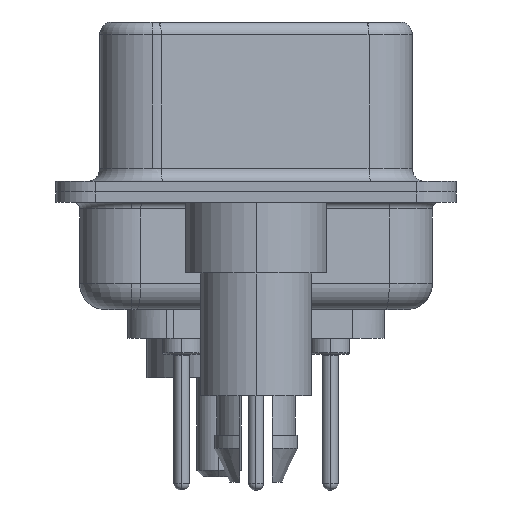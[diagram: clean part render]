
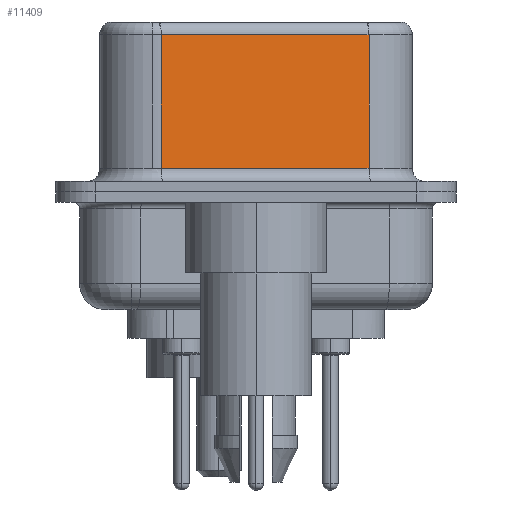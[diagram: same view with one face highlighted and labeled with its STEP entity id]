
A CAD part, left-side view. The second image highlights one B-rep face of the part: STEP entity #11409.
In plain terms, the highlighted planar face has unit normal (-0.985, -0.174, 0).
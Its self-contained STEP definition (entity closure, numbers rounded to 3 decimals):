
#6 = CARTESIAN_POINT ( 'NONE',  ( 5.132, -4.322, 6.02 ) ) ;
#261 = VECTOR ( 'NONE', #24384, 1000. ) ;
#1304 = EDGE_CURVE ( 'NONE', #33353, #19274, #29331, .T. ) ;
#1372 = EDGE_CURVE ( 'NONE', #15415, #19274, #7924, .T. ) ;
#1463 = DIRECTION ( 'NONE',  ( -0.174, 0.985, 0. ) ) ;
#1785 = CARTESIAN_POINT ( 'NONE',  ( 5.132, -4.322, 6.02 ) ) ;
#2035 = VERTEX_POINT ( 'NONE', #22724 ) ;
#3930 = CARTESIAN_POINT ( 'NONE',  ( 5.132, -4.322, 0.9 ) ) ;
#5549 = EDGE_LOOP ( 'NONE', ( #29165, #28619, #8552, #32557 ) ) ;
#7704 = VECTOR ( 'NONE', #30210, 1000. ) ;
#7924 = LINE ( 'NONE', #28003, #261 ) ;
#8552 = ORIENTED_EDGE ( 'NONE', *, *, #19182, .T. ) ;
#8731 = VECTOR ( 'NONE', #16047, 1000. ) ;
#11409 = ADVANCED_FACE ( 'NONE', ( #24887 ), #27208, .F. ) ;
#11717 = CARTESIAN_POINT ( 'NONE',  ( 5.132, -4.322, 6.52 ) ) ;
#12270 = CARTESIAN_POINT ( 'NONE',  ( 3.73, 3.628, 0.9 ) ) ;
#15415 = VERTEX_POINT ( 'NONE', #12270 ) ;
#16047 = DIRECTION ( 'NONE',  ( 0., 0., -1. ) ) ;
#16900 = DIRECTION ( 'NONE',  ( 0.985, 0.174, 0. ) ) ;
#18760 = AXIS2_PLACEMENT_3D ( 'NONE', #11717, #16900, #1463 ) ;
#18917 = CARTESIAN_POINT ( 'NONE',  ( 3.73, 3.628, 6.52 ) ) ;
#19182 = EDGE_CURVE ( 'NONE', #2035, #15415, #23547, .T. ) ;
#19274 = VERTEX_POINT ( 'NONE', #3930 ) ;
#21517 = DIRECTION ( 'NONE',  ( 0., 0., -1. ) ) ;
#21532 = EDGE_CURVE ( 'NONE', #33353, #2035, #28313, .T. ) ;
#22724 = CARTESIAN_POINT ( 'NONE',  ( 3.73, 3.628, 6.02 ) ) ;
#22733 = VECTOR ( 'NONE', #21517, 1000. ) ;
#23547 = LINE ( 'NONE', #18917, #22733 ) ;
#24384 = DIRECTION ( 'NONE',  ( 0.174, -0.985, 0. ) ) ;
#24887 = FACE_OUTER_BOUND ( 'NONE', #5549, .T. ) ;
#27208 = PLANE ( 'NONE',  #18760 ) ;
#28003 = CARTESIAN_POINT ( 'NONE',  ( 5.132, -4.322, 0.9 ) ) ;
#28313 = LINE ( 'NONE', #1785, #7704 ) ;
#28619 = ORIENTED_EDGE ( 'NONE', *, *, #21532, .T. ) ;
#29165 = ORIENTED_EDGE ( 'NONE', *, *, #1304, .F. ) ;
#29331 = LINE ( 'NONE', #30535, #8731 ) ;
#30210 = DIRECTION ( 'NONE',  ( -0.174, 0.985, 0. ) ) ;
#30535 = CARTESIAN_POINT ( 'NONE',  ( 5.132, -4.322, 6.52 ) ) ;
#32557 = ORIENTED_EDGE ( 'NONE', *, *, #1372, .T. ) ;
#33353 = VERTEX_POINT ( 'NONE', #6 ) ;
